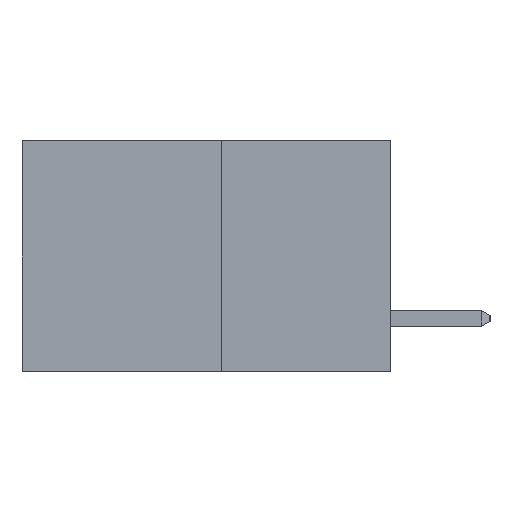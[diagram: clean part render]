
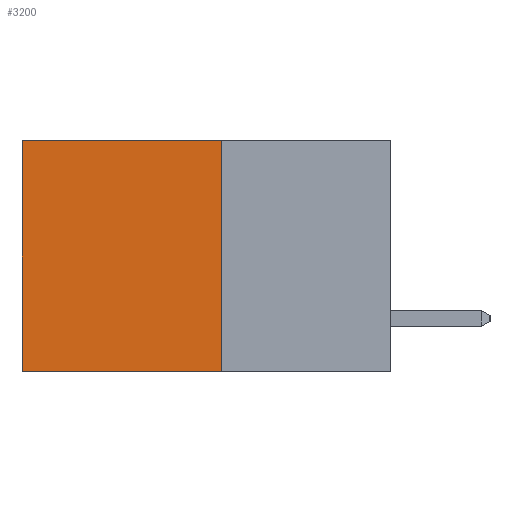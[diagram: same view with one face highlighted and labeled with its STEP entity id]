
A CAD part, left-side view. The second image highlights one B-rep face of the part: STEP entity #3200.
In plain terms, the highlighted planar face has unit normal (-1, 0, 0).
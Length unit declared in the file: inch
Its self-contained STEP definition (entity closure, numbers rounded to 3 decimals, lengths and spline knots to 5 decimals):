
#101 = DIRECTION ( 'NONE',  ( 0., 1., 0. ) ) ;
#350 = EDGE_CURVE ( 'NONE', #3575, #12961, #6244, .T. ) ;
#610 = VECTOR ( 'NONE', #12699, 39.37008 ) ;
#1046 = ORIENTED_EDGE ( 'NONE', *, *, #8559, .F. ) ;
#1457 = DIRECTION ( 'NONE',  ( 0., 0., -1. ) ) ;
#1793 = VERTEX_POINT ( 'NONE', #8884 ) ;
#2177 = EDGE_LOOP ( 'NONE', ( #9158, #1046, #11266, #4212 ) ) ;
#2298 = VECTOR ( 'NONE', #8069, 39.37008 ) ;
#3200 = ADVANCED_FACE ( 'NONE', ( #12066 ), #8579, .F. ) ;
#3575 = VERTEX_POINT ( 'NONE', #8380 ) ;
#4107 = CARTESIAN_POINT ( 'NONE',  ( 0.277, 0.59, -0.37 ) ) ;
#4212 = ORIENTED_EDGE ( 'NONE', *, *, #9996, .T. ) ;
#4497 = CARTESIAN_POINT ( 'NONE',  ( 0.277, 0.59, -0.37 ) ) ;
#4883 = CARTESIAN_POINT ( 'NONE',  ( 0.277, 0.27, 0. ) ) ;
#6244 = LINE ( 'NONE', #4107, #12466 ) ;
#6820 = AXIS2_PLACEMENT_3D ( 'NONE', #8675, #8707, #1457 ) ;
#6872 = CARTESIAN_POINT ( 'NONE',  ( 0.277, 0.27, -0.37 ) ) ;
#8069 = DIRECTION ( 'NONE',  ( 0., 0., -1. ) ) ;
#8380 = CARTESIAN_POINT ( 'NONE',  ( 0.277, 0.59, 0. ) ) ;
#8559 = EDGE_CURVE ( 'NONE', #1793, #12961, #12744, .T. ) ;
#8579 = PLANE ( 'NONE',  #6820 ) ;
#8675 = CARTESIAN_POINT ( 'NONE',  ( 0.277, 0.27, -0.37 ) ) ;
#8707 = DIRECTION ( 'NONE',  ( 1., 0., 0. ) ) ;
#8768 = VERTEX_POINT ( 'NONE', #4883 ) ;
#8884 = CARTESIAN_POINT ( 'NONE',  ( 0.277, 0.27, -0.37 ) ) ;
#8892 = LINE ( 'NONE', #14991, #2298 ) ;
#9110 = LINE ( 'NONE', #11867, #14851 ) ;
#9158 = ORIENTED_EDGE ( 'NONE', *, *, #350, .T. ) ;
#9996 = EDGE_CURVE ( 'NONE', #8768, #3575, #9110, .T. ) ;
#10468 = EDGE_CURVE ( 'NONE', #8768, #1793, #8892, .T. ) ;
#11266 = ORIENTED_EDGE ( 'NONE', *, *, #10468, .F. ) ;
#11867 = CARTESIAN_POINT ( 'NONE',  ( 0.277, 0.27, 0. ) ) ;
#12066 = FACE_OUTER_BOUND ( 'NONE', #2177, .T. ) ;
#12466 = VECTOR ( 'NONE', #13844, 39.37008 ) ;
#12699 = DIRECTION ( 'NONE',  ( 0., 1., 0. ) ) ;
#12744 = LINE ( 'NONE', #6872, #610 ) ;
#12961 = VERTEX_POINT ( 'NONE', #4497 ) ;
#13844 = DIRECTION ( 'NONE',  ( 0., 0., -1. ) ) ;
#14851 = VECTOR ( 'NONE', #101, 39.37008 ) ;
#14991 = CARTESIAN_POINT ( 'NONE',  ( 0.277, 0.27, -0.37 ) ) ;
